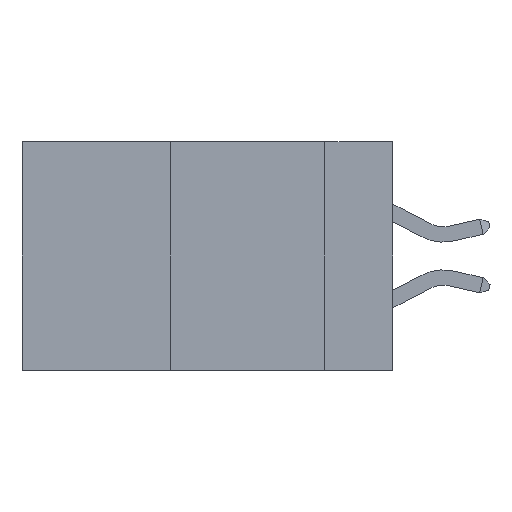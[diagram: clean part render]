
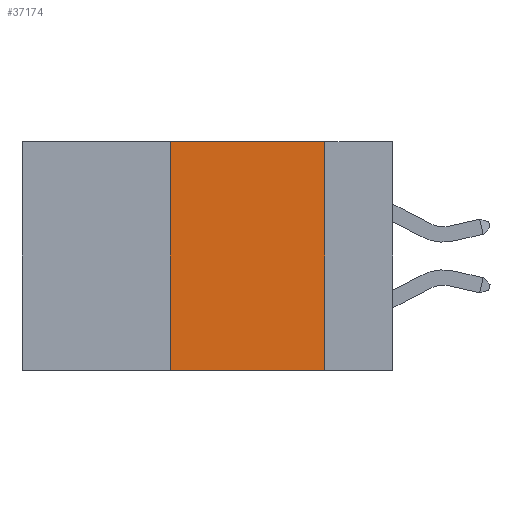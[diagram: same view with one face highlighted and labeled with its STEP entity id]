
A CAD part, left-side view. The second image highlights one B-rep face of the part: STEP entity #37174.
In plain terms, the highlighted planar face has unit normal (-1, 0, 0).
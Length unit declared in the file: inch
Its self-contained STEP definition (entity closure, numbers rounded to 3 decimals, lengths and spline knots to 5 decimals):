
#944 = CARTESIAN_POINT ( 'NONE',  ( 0., 0.6, -0.37 ) ) ;
#1908 = CARTESIAN_POINT ( 'NONE',  ( 0., 0.11, 0. ) ) ;
#3561 = EDGE_CURVE ( 'NONE', #25355, #6773, #30367, .T. ) ;
#4123 = EDGE_CURVE ( 'NONE', #25355, #34806, #32120, .T. ) ;
#4323 = ORIENTED_EDGE ( 'NONE', *, *, #31385, .F. ) ;
#5011 = DIRECTION ( 'NONE',  ( 0., 0., -1. ) ) ;
#6773 = VERTEX_POINT ( 'NONE', #21631 ) ;
#9269 = VECTOR ( 'NONE', #16752, 39.37008 ) ;
#9869 = EDGE_CURVE ( 'NONE', #13629, #34806, #19332, .T. ) ;
#11727 = VECTOR ( 'NONE', #18822, 39.37008 ) ;
#13424 = CARTESIAN_POINT ( 'NONE',  ( 0., 0.11, -0.37 ) ) ;
#13615 = ORIENTED_EDGE ( 'NONE', *, *, #9869, .F. ) ;
#13629 = VERTEX_POINT ( 'NONE', #21176 ) ;
#16752 = DIRECTION ( 'NONE',  ( 0., -1., 0. ) ) ;
#18822 = DIRECTION ( 'NONE',  ( 0., 0., -1. ) ) ;
#18944 = PLANE ( 'NONE',  #31784 ) ;
#19332 = LINE ( 'NONE', #1908, #11727 ) ;
#21176 = CARTESIAN_POINT ( 'NONE',  ( 0., 0.11, 0. ) ) ;
#21308 = EDGE_LOOP ( 'NONE', ( #13615, #4323, #29241, #28712 ) ) ;
#21631 = CARTESIAN_POINT ( 'NONE',  ( 0., 0.36, 0. ) ) ;
#23576 = CARTESIAN_POINT ( 'NONE',  ( 0., 0.36, -0.37 ) ) ;
#24449 = VECTOR ( 'NONE', #26771, 39.37008 ) ;
#25355 = VERTEX_POINT ( 'NONE', #23576 ) ;
#26500 = CARTESIAN_POINT ( 'NONE',  ( 0., 0.36, 0. ) ) ;
#26771 = DIRECTION ( 'NONE',  ( 0., -1., 0. ) ) ;
#27777 = CARTESIAN_POINT ( 'NONE',  ( 0., 0.6, 0. ) ) ;
#27840 = CARTESIAN_POINT ( 'NONE',  ( 0., 0.6, 0. ) ) ;
#28192 = DIRECTION ( 'NONE',  ( 0., 0., 1. ) ) ;
#28712 = ORIENTED_EDGE ( 'NONE', *, *, #4123, .T. ) ;
#29241 = ORIENTED_EDGE ( 'NONE', *, *, #3561, .F. ) ;
#30028 = FACE_OUTER_BOUND ( 'NONE', #21308, .T. ) ;
#30367 = LINE ( 'NONE', #26500, #33970 ) ;
#30916 = DIRECTION ( 'NONE',  ( 1., 0., 0. ) ) ;
#31385 = EDGE_CURVE ( 'NONE', #6773, #13629, #31807, .T. ) ;
#31784 = AXIS2_PLACEMENT_3D ( 'NONE', #27777, #30916, #5011 ) ;
#31807 = LINE ( 'NONE', #27840, #9269 ) ;
#32120 = LINE ( 'NONE', #944, #24449 ) ;
#33970 = VECTOR ( 'NONE', #28192, 39.37008 ) ;
#34806 = VERTEX_POINT ( 'NONE', #13424 ) ;
#37174 = ADVANCED_FACE ( 'NONE', ( #30028 ), #18944, .F. ) ;
